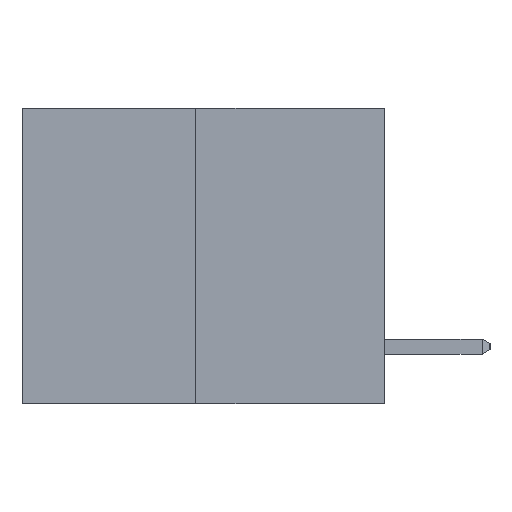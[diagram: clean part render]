
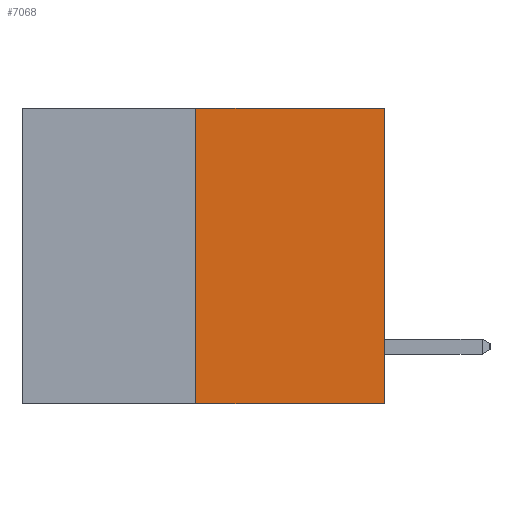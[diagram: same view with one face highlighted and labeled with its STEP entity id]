
A CAD part, left-side view. The second image highlights one B-rep face of the part: STEP entity #7068.
In plain terms, the highlighted planar face has unit normal (-1, 0, 0).
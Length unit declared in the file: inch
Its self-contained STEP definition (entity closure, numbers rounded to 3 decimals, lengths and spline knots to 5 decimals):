
#289 = EDGE_CURVE ( 'NONE', #9427, #4416, #11525, .T. ) ;
#567 = DIRECTION ( 'NONE',  ( 0., -1., 0. ) ) ;
#822 = DIRECTION ( 'NONE',  ( 0., 0., 1. ) ) ;
#913 = PLANE ( 'NONE',  #6415 ) ;
#1841 = EDGE_CURVE ( 'NONE', #5157, #2672, #9901, .T. ) ;
#1923 = LINE ( 'NONE', #7211, #6540 ) ;
#2607 = DIRECTION ( 'NONE',  ( 0., 0., 1. ) ) ;
#2633 = CARTESIAN_POINT ( 'NONE',  ( 0., 0., 0. ) ) ;
#2672 = VERTEX_POINT ( 'NONE', #2633 ) ;
#2738 = ORIENTED_EDGE ( 'NONE', *, *, #289, .F. ) ;
#2794 = DIRECTION ( 'NONE',  ( 1., 0., 0. ) ) ;
#2860 = ORIENTED_EDGE ( 'NONE', *, *, #5402, .T. ) ;
#3053 = CARTESIAN_POINT ( 'NONE',  ( 0., 0.312, -0.49 ) ) ;
#3377 = VECTOR ( 'NONE', #2607, 39.37008 ) ;
#3584 = EDGE_LOOP ( 'NONE', ( #2738, #2860, #8967, #10273 ) ) ;
#4416 = VERTEX_POINT ( 'NONE', #11042 ) ;
#4561 = DIRECTION ( 'NONE',  ( 0., -1., 0. ) ) ;
#4631 = CARTESIAN_POINT ( 'NONE',  ( 0., 0.6, 0. ) ) ;
#5157 = VERTEX_POINT ( 'NONE', #5670 ) ;
#5402 = EDGE_CURVE ( 'NONE', #9427, #5157, #8788, .T. ) ;
#5670 = CARTESIAN_POINT ( 'NONE',  ( 0., 0., -0.49 ) ) ;
#6322 = VECTOR ( 'NONE', #567, 39.37008 ) ;
#6415 = AXIS2_PLACEMENT_3D ( 'NONE', #4631, #2794, #7310 ) ;
#6444 = CARTESIAN_POINT ( 'NONE',  ( 0., 0.312, -0.49 ) ) ;
#6540 = VECTOR ( 'NONE', #4561, 39.37008 ) ;
#7035 = CARTESIAN_POINT ( 'NONE',  ( 0., 0., 0. ) ) ;
#7068 = ADVANCED_FACE ( 'NONE', ( #10160 ), #913, .F. ) ;
#7211 = CARTESIAN_POINT ( 'NONE',  ( 0., 0.6, 0. ) ) ;
#7310 = DIRECTION ( 'NONE',  ( 0., 0., -1. ) ) ;
#7599 = EDGE_CURVE ( 'NONE', #4416, #2672, #1923, .T. ) ;
#8631 = VECTOR ( 'NONE', #822, 39.37008 ) ;
#8788 = LINE ( 'NONE', #11578, #6322 ) ;
#8967 = ORIENTED_EDGE ( 'NONE', *, *, #1841, .T. ) ;
#9427 = VERTEX_POINT ( 'NONE', #3053 ) ;
#9901 = LINE ( 'NONE', #7035, #3377 ) ;
#10160 = FACE_OUTER_BOUND ( 'NONE', #3584, .T. ) ;
#10273 = ORIENTED_EDGE ( 'NONE', *, *, #7599, .F. ) ;
#11042 = CARTESIAN_POINT ( 'NONE',  ( 0., 0.312, 0. ) ) ;
#11525 = LINE ( 'NONE', #6444, #8631 ) ;
#11578 = CARTESIAN_POINT ( 'NONE',  ( 0., 0.6, -0.49 ) ) ;
